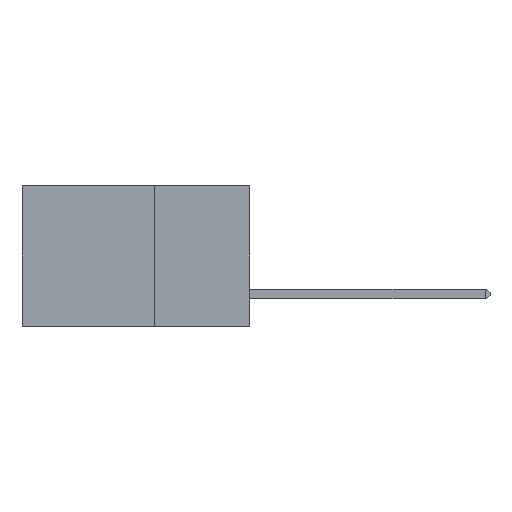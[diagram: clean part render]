
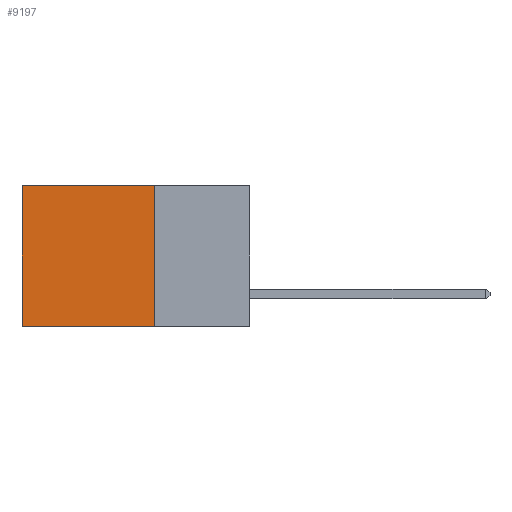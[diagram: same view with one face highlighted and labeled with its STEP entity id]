
A CAD part, left-side view. The second image highlights one B-rep face of the part: STEP entity #9197.
In plain terms, the highlighted planar face has unit normal (-1, 0, 0).
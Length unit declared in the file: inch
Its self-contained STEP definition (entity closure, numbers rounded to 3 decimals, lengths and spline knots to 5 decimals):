
#437 = CARTESIAN_POINT ( 'NONE',  ( 0.2875, 0.25, 0. ) ) ;
#627 = EDGE_CURVE ( 'NONE', #7736, #793, #10147, .T. ) ;
#793 = VERTEX_POINT ( 'NONE', #13172 ) ;
#1168 = EDGE_CURVE ( 'NONE', #2502, #2471, #13209, .T. ) ;
#1559 = EDGE_LOOP ( 'NONE', ( #8463, #9544, #7170, #14013 ) ) ;
#2471 = VERTEX_POINT ( 'NONE', #9783 ) ;
#2502 = VERTEX_POINT ( 'NONE', #437 ) ;
#5024 = CARTESIAN_POINT ( 'NONE',  ( 0.2875, 0.25, -0.37 ) ) ;
#5143 = CARTESIAN_POINT ( 'NONE',  ( 0.2875, 0.25, -0.37 ) ) ;
#5633 = PLANE ( 'NONE',  #14711 ) ;
#6331 = VECTOR ( 'NONE', #14429, 39.37008 ) ;
#6581 = VECTOR ( 'NONE', #8009, 39.37008 ) ;
#6809 = DIRECTION ( 'NONE',  ( 1., 0., 0. ) ) ;
#6810 = DIRECTION ( 'NONE',  ( 0., 1., 0. ) ) ;
#7170 = ORIENTED_EDGE ( 'NONE', *, *, #13890, .F. ) ;
#7649 = VECTOR ( 'NONE', #12918, 39.37008 ) ;
#7736 = VERTEX_POINT ( 'NONE', #5143 ) ;
#8009 = DIRECTION ( 'NONE',  ( 0., 0., -1. ) ) ;
#8463 = ORIENTED_EDGE ( 'NONE', *, *, #12263, .T. ) ;
#9197 = ADVANCED_FACE ( 'NONE', ( #9972 ), #5633, .F. ) ;
#9544 = ORIENTED_EDGE ( 'NONE', *, *, #627, .F. ) ;
#9620 = LINE ( 'NONE', #12399, #6581 ) ;
#9783 = CARTESIAN_POINT ( 'NONE',  ( 0.2875, 0.6, 0. ) ) ;
#9808 = VECTOR ( 'NONE', #6810, 39.37008 ) ;
#9972 = FACE_OUTER_BOUND ( 'NONE', #1559, .T. ) ;
#9987 = CARTESIAN_POINT ( 'NONE',  ( 0.2875, 0.25, 0. ) ) ;
#10147 = LINE ( 'NONE', #5024, #9808 ) ;
#12263 = EDGE_CURVE ( 'NONE', #2471, #793, #12300, .T. ) ;
#12300 = LINE ( 'NONE', #13318, #6331 ) ;
#12399 = CARTESIAN_POINT ( 'NONE',  ( 0.2875, 0.25, 0. ) ) ;
#12918 = DIRECTION ( 'NONE',  ( 0., 1., 0. ) ) ;
#13172 = CARTESIAN_POINT ( 'NONE',  ( 0.2875, 0.6, -0.37 ) ) ;
#13209 = LINE ( 'NONE', #9987, #7649 ) ;
#13318 = CARTESIAN_POINT ( 'NONE',  ( 0.2875, 0.6, 0. ) ) ;
#13490 = CARTESIAN_POINT ( 'NONE',  ( 0.2875, 0.25, 0. ) ) ;
#13890 = EDGE_CURVE ( 'NONE', #2502, #7736, #9620, .T. ) ;
#14013 = ORIENTED_EDGE ( 'NONE', *, *, #1168, .T. ) ;
#14429 = DIRECTION ( 'NONE',  ( 0., 0., -1. ) ) ;
#14602 = DIRECTION ( 'NONE',  ( 0., 0., -1. ) ) ;
#14711 = AXIS2_PLACEMENT_3D ( 'NONE', #13490, #6809, #14602 ) ;
